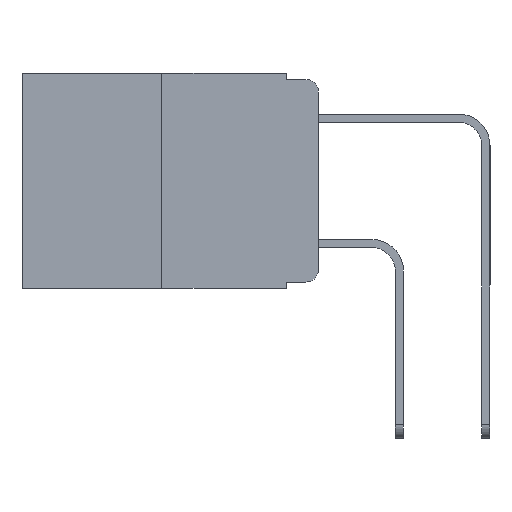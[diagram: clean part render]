
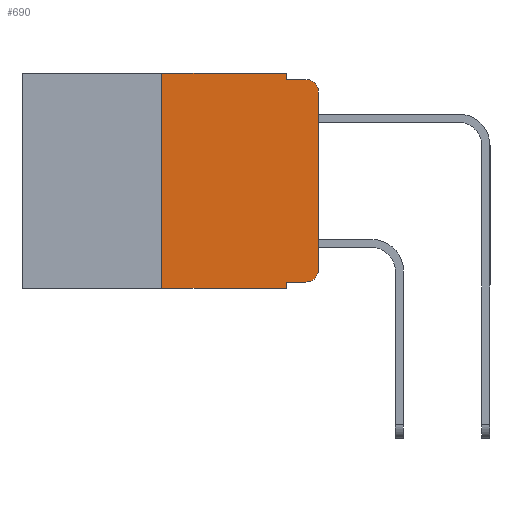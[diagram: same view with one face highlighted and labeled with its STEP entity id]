
A CAD part, left-side view. The second image highlights one B-rep face of the part: STEP entity #690.
In plain terms, the highlighted planar face has unit normal (-1, 0, 0).
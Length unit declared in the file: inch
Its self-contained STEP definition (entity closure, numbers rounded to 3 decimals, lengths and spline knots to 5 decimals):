
#255 = LINE ( 'NONE', #15014, #7493 ) ;
#277 = LINE ( 'NONE', #684, #11154 ) ;
#684 = CARTESIAN_POINT ( 'NONE',  ( 0., 0.051, -0.333 ) ) ;
#690 = ADVANCED_FACE ( 'NONE', ( #10428 ), #7368, .F. ) ;
#724 = CARTESIAN_POINT ( 'NONE',  ( 0., 0.02, -0.333 ) ) ;
#927 = EDGE_CURVE ( 'NONE', #4674, #4717, #1388, .T. ) ;
#1101 = CARTESIAN_POINT ( 'NONE',  ( 0., 0.25, 0. ) ) ;
#1222 = CARTESIAN_POINT ( 'NONE',  ( 0., 0., -0.313 ) ) ;
#1234 = VERTEX_POINT ( 'NONE', #13553 ) ;
#1364 = VERTEX_POINT ( 'NONE', #1222 ) ;
#1388 = LINE ( 'NONE', #13095, #15813 ) ;
#1686 = EDGE_CURVE ( 'NONE', #16872, #7717, #255, .T. ) ;
#1811 = CARTESIAN_POINT ( 'NONE',  ( 0., 0.051, 0. ) ) ;
#1968 = DIRECTION ( 'NONE',  ( -1., 0., 0. ) ) ;
#2208 = ORIENTED_EDGE ( 'NONE', *, *, #17568, .F. ) ;
#2256 = DIRECTION ( 'NONE',  ( 0., 0., -1. ) ) ;
#2335 = CARTESIAN_POINT ( 'NONE',  ( 0., 0.473, 0. ) ) ;
#2609 = AXIS2_PLACEMENT_3D ( 'NONE', #2335, #11679, #11498 ) ;
#2765 = CARTESIAN_POINT ( 'NONE',  ( 0., 0.25, -0.343 ) ) ;
#2812 = LINE ( 'NONE', #9141, #17136 ) ;
#3353 = ORIENTED_EDGE ( 'NONE', *, *, #927, .T. ) ;
#3666 = DIRECTION ( 'NONE',  ( -1., 0., 0. ) ) ;
#3791 = CARTESIAN_POINT ( 'NONE',  ( 0., 0.02, -0.01 ) ) ;
#3929 = VERTEX_POINT ( 'NONE', #16376 ) ;
#4667 = ORIENTED_EDGE ( 'NONE', *, *, #7068, .F. ) ;
#4674 = VERTEX_POINT ( 'NONE', #2765 ) ;
#4717 = VERTEX_POINT ( 'NONE', #7074 ) ;
#4985 = DIRECTION ( 'NONE',  ( 0., 0., -1. ) ) ;
#5112 = VECTOR ( 'NONE', #9054, 39.37008 ) ;
#5134 = CARTESIAN_POINT ( 'NONE',  ( 0., 0.051, 0. ) ) ;
#5159 = VERTEX_POINT ( 'NONE', #3791 ) ;
#5908 = LINE ( 'NONE', #5134, #12369 ) ;
#6212 = CARTESIAN_POINT ( 'NONE',  ( 0., 0.25, 0. ) ) ;
#6550 = CIRCLE ( 'NONE', #14036, 0.02 ) ;
#7068 = EDGE_CURVE ( 'NONE', #9339, #5159, #13802, .T. ) ;
#7074 = CARTESIAN_POINT ( 'NONE',  ( 0., 0.051, -0.343 ) ) ;
#7309 = ORIENTED_EDGE ( 'NONE', *, *, #1686, .F. ) ;
#7363 = EDGE_LOOP ( 'NONE', ( #16354, #18085, #4667, #2208, #7309, #9067, #3353, #11435, #15567, #9977 ) ) ;
#7368 = PLANE ( 'NONE',  #2609 ) ;
#7493 = VECTOR ( 'NONE', #15561, 39.37008 ) ;
#7597 = DIRECTION ( 'NONE',  ( 0., -1., 0. ) ) ;
#7609 = LINE ( 'NONE', #1101, #10826 ) ;
#7717 = VERTEX_POINT ( 'NONE', #1811 ) ;
#8210 = DIRECTION ( 'NONE',  ( 0., 0., 1. ) ) ;
#9049 = EDGE_CURVE ( 'NONE', #10334, #1364, #15177, .T. ) ;
#9054 = DIRECTION ( 'NONE',  ( 0., 0., 1. ) ) ;
#9067 = ORIENTED_EDGE ( 'NONE', *, *, #9293, .F. ) ;
#9141 = CARTESIAN_POINT ( 'NONE',  ( 0., 0.051, 0. ) ) ;
#9293 = EDGE_CURVE ( 'NONE', #4674, #16872, #7609, .T. ) ;
#9339 = VERTEX_POINT ( 'NONE', #13796 ) ;
#9977 = ORIENTED_EDGE ( 'NONE', *, *, #9049, .T. ) ;
#10126 = VECTOR ( 'NONE', #7597, 39.37008 ) ;
#10334 = VERTEX_POINT ( 'NONE', #724 ) ;
#10372 = CARTESIAN_POINT ( 'NONE',  ( 0., 0.02, -0.03 ) ) ;
#10428 = FACE_OUTER_BOUND ( 'NONE', #7363, .T. ) ;
#10519 = DIRECTION ( 'NONE',  ( 0., -1., 0. ) ) ;
#10826 = VECTOR ( 'NONE', #8210, 39.37008 ) ;
#11154 = VECTOR ( 'NONE', #10519, 39.37008 ) ;
#11435 = ORIENTED_EDGE ( 'NONE', *, *, #16996, .F. ) ;
#11498 = DIRECTION ( 'NONE',  ( 0., 0., -1. ) ) ;
#11679 = DIRECTION ( 'NONE',  ( 1., 0., 0. ) ) ;
#11737 = DIRECTION ( 'NONE',  ( 0., 0., -1. ) ) ;
#11893 = AXIS2_PLACEMENT_3D ( 'NONE', #11974, #3666, #13371 ) ;
#11974 = CARTESIAN_POINT ( 'NONE',  ( 0., 0.02, -0.313 ) ) ;
#12369 = VECTOR ( 'NONE', #2256, 39.37008 ) ;
#12868 = LINE ( 'NONE', #15889, #5112 ) ;
#13095 = CARTESIAN_POINT ( 'NONE',  ( 0., 0.473, -0.343 ) ) ;
#13371 = DIRECTION ( 'NONE',  ( 0., 0., -1. ) ) ;
#13553 = CARTESIAN_POINT ( 'NONE',  ( 0., 0.051, -0.333 ) ) ;
#13574 = EDGE_CURVE ( 'NONE', #3929, #5159, #6550, .T. ) ;
#13796 = CARTESIAN_POINT ( 'NONE',  ( 0., 0.051, -0.01 ) ) ;
#13802 = LINE ( 'NONE', #15851, #10126 ) ;
#14036 = AXIS2_PLACEMENT_3D ( 'NONE', #10372, #1968, #11737 ) ;
#14078 = DIRECTION ( 'NONE',  ( 0., -1., 0. ) ) ;
#15014 = CARTESIAN_POINT ( 'NONE',  ( 0., 0.473, 0. ) ) ;
#15084 = EDGE_CURVE ( 'NONE', #1364, #3929, #12868, .T. ) ;
#15156 = EDGE_CURVE ( 'NONE', #1234, #10334, #277, .T. ) ;
#15177 = CIRCLE ( 'NONE', #11893, 0.02 ) ;
#15561 = DIRECTION ( 'NONE',  ( 0., -1., 0. ) ) ;
#15567 = ORIENTED_EDGE ( 'NONE', *, *, #15156, .T. ) ;
#15813 = VECTOR ( 'NONE', #14078, 39.37008 ) ;
#15851 = CARTESIAN_POINT ( 'NONE',  ( 0., 0.051, -0.01 ) ) ;
#15889 = CARTESIAN_POINT ( 'NONE',  ( 0., 0., 0. ) ) ;
#16354 = ORIENTED_EDGE ( 'NONE', *, *, #15084, .T. ) ;
#16376 = CARTESIAN_POINT ( 'NONE',  ( 0., 0., -0.03 ) ) ;
#16872 = VERTEX_POINT ( 'NONE', #6212 ) ;
#16996 = EDGE_CURVE ( 'NONE', #1234, #4717, #5908, .T. ) ;
#17136 = VECTOR ( 'NONE', #4985, 39.37008 ) ;
#17568 = EDGE_CURVE ( 'NONE', #7717, #9339, #2812, .T. ) ;
#18085 = ORIENTED_EDGE ( 'NONE', *, *, #13574, .T. ) ;
